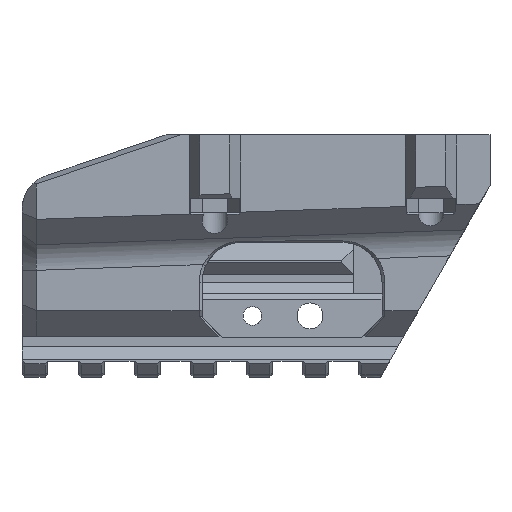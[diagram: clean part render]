
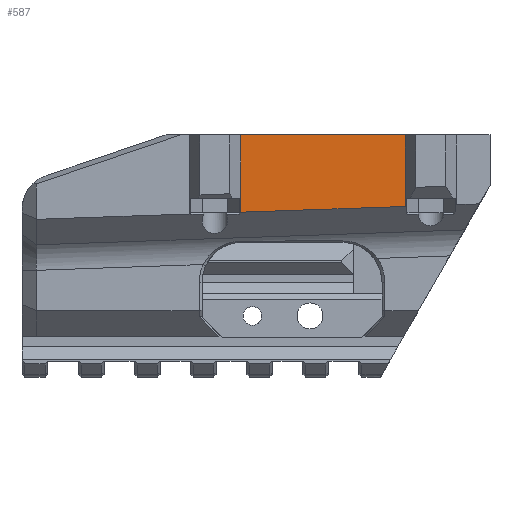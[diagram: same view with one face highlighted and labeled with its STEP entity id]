
A CAD part, top view. The second image highlights one B-rep face of the part: STEP entity #587.
In plain terms, the highlighted planar face has unit normal (0, 0, 1).
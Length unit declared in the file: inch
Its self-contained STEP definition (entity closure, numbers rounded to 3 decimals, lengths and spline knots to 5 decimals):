
#152 = EDGE_CURVE ( 'NONE', #4613, #10154, #253, .T. ) ;
#253 = LINE ( 'NONE', #7216, #12618 ) ;
#587 = ADVANCED_FACE ( 'NONE', ( #14538 ), #6161, .T. ) ;
#1774 = DIRECTION ( 'NONE',  ( -1., 0., 0. ) ) ;
#1894 = ORIENTED_EDGE ( 'NONE', *, *, #9794, .T. ) ;
#2281 = VERTEX_POINT ( 'NONE', #8425 ) ;
#3091 = CARTESIAN_POINT ( 'NONE',  ( 1., 0., 0.94882 ) ) ;
#3951 = CARTESIAN_POINT ( 'NONE',  ( 2.66102, 0., 0.94882 ) ) ;
#4613 = VERTEX_POINT ( 'NONE', #12529 ) ;
#4856 = EDGE_CURVE ( 'NONE', #4613, #11539, #10076, .T. ) ;
#4982 = CARTESIAN_POINT ( 'NONE',  ( 3.02175, -0.48433, 0.94882 ) ) ;
#5199 = LINE ( 'NONE', #3951, #11912 ) ;
#5321 = CARTESIAN_POINT ( 'NONE',  ( 2.66102, -0.49692, 0.94882 ) ) ;
#5934 = DIRECTION ( 'NONE',  ( 0., 0., 1. ) ) ;
#6161 = PLANE ( 'NONE',  #10011 ) ;
#6289 = DIRECTION ( 'NONE',  ( 0., 1., 0. ) ) ;
#6382 = VECTOR ( 'NONE', #9770, 39.37008 ) ;
#6513 = ORIENTED_EDGE ( 'NONE', *, *, #11147, .T. ) ;
#6730 = ORIENTED_EDGE ( 'NONE', *, *, #152, .F. ) ;
#6813 = EDGE_LOOP ( 'NONE', ( #7091, #6513, #1894, #6730 ) ) ;
#7091 = ORIENTED_EDGE ( 'NONE', *, *, #4856, .T. ) ;
#7216 = CARTESIAN_POINT ( 'NONE',  ( 1.51898, 0., 0.94882 ) ) ;
#8425 = CARTESIAN_POINT ( 'NONE',  ( 2.66102, 0., 0.94882 ) ) ;
#9770 = DIRECTION ( 'NONE',  ( 0.999, 0.035, 0. ) ) ;
#9794 = EDGE_CURVE ( 'NONE', #2281, #10154, #11391, .T. ) ;
#10011 = AXIS2_PLACEMENT_3D ( 'NONE', #14387, #5934, #10946 ) ;
#10076 = LINE ( 'NONE', #4982, #6382 ) ;
#10154 = VERTEX_POINT ( 'NONE', #12795 ) ;
#10560 = VECTOR ( 'NONE', #1774, 39.37008 ) ;
#10946 = DIRECTION ( 'NONE',  ( 1., 0., 0. ) ) ;
#11147 = EDGE_CURVE ( 'NONE', #11539, #2281, #5199, .T. ) ;
#11391 = LINE ( 'NONE', #3091, #10560 ) ;
#11539 = VERTEX_POINT ( 'NONE', #5321 ) ;
#11912 = VECTOR ( 'NONE', #6289, 39.37008 ) ;
#12529 = CARTESIAN_POINT ( 'NONE',  ( 1.51898, -0.5368, 0.94882 ) ) ;
#12618 = VECTOR ( 'NONE', #14329, 39.37008 ) ;
#12795 = CARTESIAN_POINT ( 'NONE',  ( 1.51898, 0., 0.94882 ) ) ;
#14329 = DIRECTION ( 'NONE',  ( 0., 1., 0. ) ) ;
#14387 = CARTESIAN_POINT ( 'NONE',  ( 0., 0., 0.94882 ) ) ;
#14538 = FACE_OUTER_BOUND ( 'NONE', #6813, .T. ) ;
